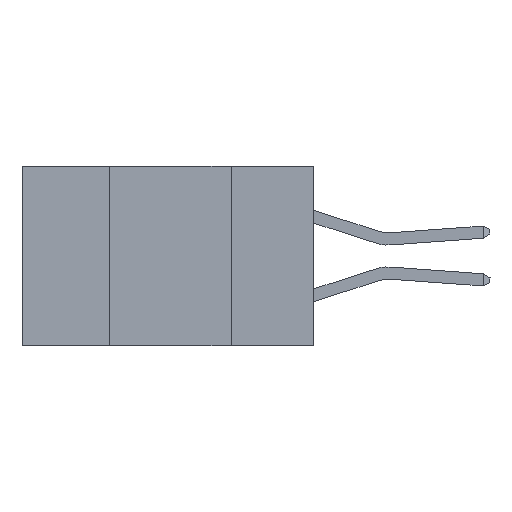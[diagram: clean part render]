
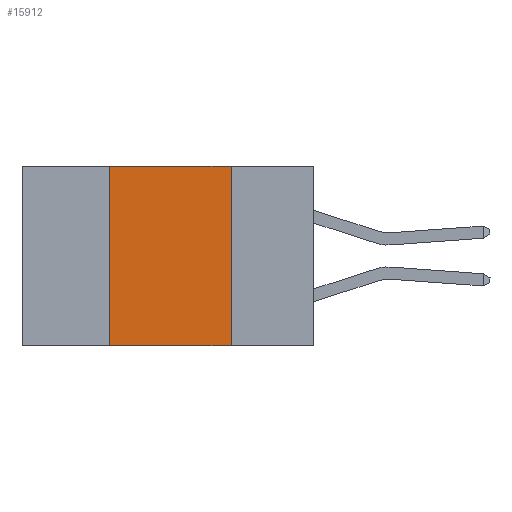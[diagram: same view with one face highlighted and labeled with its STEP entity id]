
A CAD part, left-side view. The second image highlights one B-rep face of the part: STEP entity #15912.
In plain terms, the highlighted planar face has unit normal (-1, 0, 0).
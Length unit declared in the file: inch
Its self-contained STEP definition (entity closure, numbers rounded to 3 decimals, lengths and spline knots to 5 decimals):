
#1553 = EDGE_CURVE ( 'NONE', #3119, #4310, #23669, .T. ) ;
#3100 = EDGE_CURVE ( 'NONE', #3119, #24177, #18466, .T. ) ;
#3119 = VERTEX_POINT ( 'NONE', #24426 ) ;
#3523 = CARTESIAN_POINT ( 'NONE',  ( 0., 0.42, 0. ) ) ;
#3545 = ORIENTED_EDGE ( 'NONE', *, *, #3100, .T. ) ;
#4053 = DIRECTION ( 'NONE',  ( 0., 0., 1. ) ) ;
#4310 = VERTEX_POINT ( 'NONE', #3523 ) ;
#4994 = ORIENTED_EDGE ( 'NONE', *, *, #14264, .F. ) ;
#6419 = ORIENTED_EDGE ( 'NONE', *, *, #1553, .F. ) ;
#6537 = LINE ( 'NONE', #21710, #15012 ) ;
#7360 = AXIS2_PLACEMENT_3D ( 'NONE', #20847, #9006, #16782 ) ;
#7995 = VECTOR ( 'NONE', #18587, 39.37008 ) ;
#8981 = VECTOR ( 'NONE', #4053, 39.37008 ) ;
#9006 = DIRECTION ( 'NONE',  ( 1., 0., 0. ) ) ;
#9155 = LINE ( 'NONE', #20872, #9349 ) ;
#9349 = VECTOR ( 'NONE', #15785, 39.37008 ) ;
#11162 = FACE_OUTER_BOUND ( 'NONE', #16698, .T. ) ;
#11406 = EDGE_CURVE ( 'NONE', #4310, #14459, #6537, .T. ) ;
#12738 = ORIENTED_EDGE ( 'NONE', *, *, #11406, .F. ) ;
#14264 = EDGE_CURVE ( 'NONE', #14459, #24177, #9155, .T. ) ;
#14459 = VERTEX_POINT ( 'NONE', #24020 ) ;
#15012 = VECTOR ( 'NONE', #21822, 39.37008 ) ;
#15785 = DIRECTION ( 'NONE',  ( 0., 0., -1. ) ) ;
#15912 = ADVANCED_FACE ( 'NONE', ( #11162 ), #16904, .F. ) ;
#16065 = CARTESIAN_POINT ( 'NONE',  ( 0., 0.42, 0. ) ) ;
#16698 = EDGE_LOOP ( 'NONE', ( #4994, #12738, #6419, #3545 ) ) ;
#16782 = DIRECTION ( 'NONE',  ( 0., 0., -1. ) ) ;
#16904 = PLANE ( 'NONE',  #7360 ) ;
#18466 = LINE ( 'NONE', #22258, #7995 ) ;
#18587 = DIRECTION ( 'NONE',  ( 0., -1., 0. ) ) ;
#20290 = CARTESIAN_POINT ( 'NONE',  ( 0., 0.17, -0.37 ) ) ;
#20847 = CARTESIAN_POINT ( 'NONE',  ( 0., 0.6, 0. ) ) ;
#20872 = CARTESIAN_POINT ( 'NONE',  ( 0., 0.17, 0. ) ) ;
#21710 = CARTESIAN_POINT ( 'NONE',  ( 0., 0.6, 0. ) ) ;
#21822 = DIRECTION ( 'NONE',  ( 0., -1., 0. ) ) ;
#22258 = CARTESIAN_POINT ( 'NONE',  ( 0., 0.6, -0.37 ) ) ;
#23669 = LINE ( 'NONE', #16065, #8981 ) ;
#24020 = CARTESIAN_POINT ( 'NONE',  ( 0., 0.17, 0. ) ) ;
#24177 = VERTEX_POINT ( 'NONE', #20290 ) ;
#24426 = CARTESIAN_POINT ( 'NONE',  ( 0., 0.42, -0.37 ) ) ;
